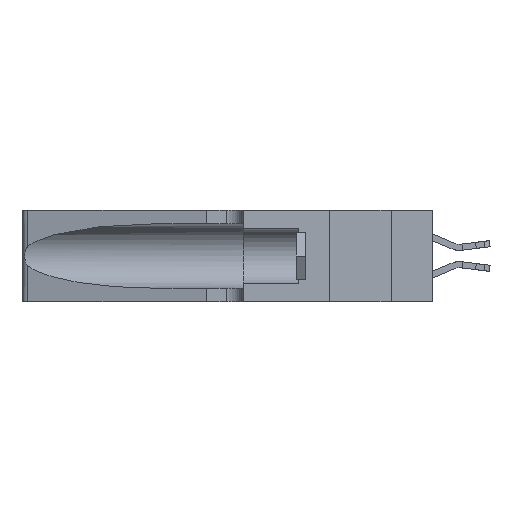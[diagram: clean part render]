
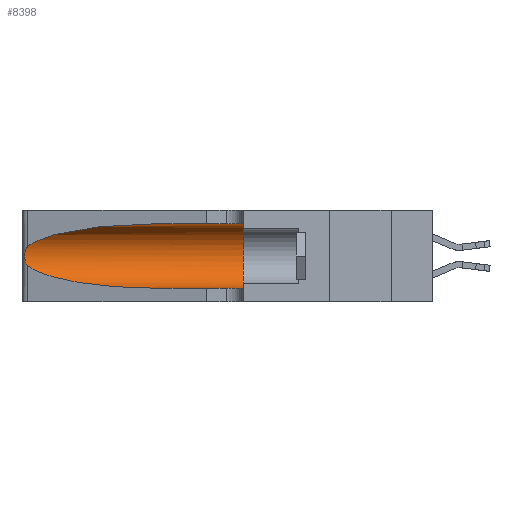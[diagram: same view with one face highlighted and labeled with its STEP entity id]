
A CAD part, left-side view. The second image highlights one B-rep face of the part: STEP entity #8398.
In plain terms, the highlighted cylindrical face has radius 3.308 mm (diameter 6.617 mm), a partial arc.
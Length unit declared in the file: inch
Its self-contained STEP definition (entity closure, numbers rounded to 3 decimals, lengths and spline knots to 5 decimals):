
#707 = CARTESIAN_POINT ( 'NONE',  ( 0.2373, 1.15595, 0.28018 ) ) ;
#922 = VECTOR ( 'NONE', #23108, 39.37008 ) ;
#1194 = CARTESIAN_POINT ( 'NONE',  ( 0.25487, 1.22718, 0.14631 ) ) ;
#1279 = DIRECTION ( 'NONE',  ( 0., 0., 1. ) ) ;
#1360 = ORIENTED_EDGE ( 'NONE', *, *, #14888, .F. ) ;
#1489 = CARTESIAN_POINT ( 'NONE',  ( 0.18966, 0.96281, 0.05475 ) ) ;
#2453 = LINE ( 'NONE', #9547, #922 ) ;
#2675 = CARTESIAN_POINT ( 'NONE',  ( 0.18966, 0.96281, 0.31525 ) ) ;
#3055 = EDGE_CURVE ( 'NONE', #12755, #5751, #14692, .T. ) ;
#3544 = CARTESIAN_POINT ( 'NONE',  ( 0.2373, 1.15595, 0.08982 ) ) ;
#4794 = DIRECTION ( 'NONE',  ( 0., 0., -1. ) ) ;
#4878 = CARTESIAN_POINT ( 'NONE',  ( 0.26075, 1.23896, 0.19203 ) ) ;
#4987 = CARTESIAN_POINT ( 'NONE',  ( 0.1305, 0.72297, 0.05475 ) ) ;
#5050 = CARTESIAN_POINT ( 'NONE',  ( 0.25854, 1.2359, 0.20912 ) ) ;
#5258 = EDGE_CURVE ( 'NONE', #9538, #23373, #2453, .T. ) ;
#5751 = VERTEX_POINT ( 'NONE', #22808 ) ;
#6125 = DIRECTION ( 'NONE',  ( 0., -1., 0. ) ) ;
#6183 = AXIS2_PLACEMENT_3D ( 'NONE', #6926, #8878, #1279 ) ;
#6446 = CARTESIAN_POINT ( 'NONE',  ( 0.1305, 0.35, 0.31525 ) ) ;
#6926 = CARTESIAN_POINT ( 'NONE',  ( 0.1305, 0.35, 0.185 ) ) ;
#7015 = CARTESIAN_POINT ( 'NONE',  ( 0.25856, 1.23593, 0.16098 ) ) ;
#7385 = CARTESIAN_POINT ( 'NONE',  ( 0.1305, 0.72297, 0.05475 ) ) ;
#7929 = CARTESIAN_POINT ( 'NONE',  ( 0.25487, 1.22718, 0.14631 ) ) ;
#8147 = CARTESIAN_POINT ( 'NONE',  ( 0.1305, 0.35, 0.05475 ) ) ;
#8299 = ORIENTED_EDGE ( 'NONE', *, *, #3055, .T. ) ;
#8398 = ADVANCED_FACE ( 'NONE', ( #16688 ), #8464, .F. ) ;
#8464 = CYLINDRICAL_SURFACE ( 'NONE', #13961, 0.13025 ) ;
#8497 = EDGE_CURVE ( 'NONE', #5751, #16210, #12018, .T. ) ;
#8878 = DIRECTION ( 'NONE',  ( 0., 1., 0. ) ) ;
#8970 = CARTESIAN_POINT ( 'NONE',  ( 0.25487, 1.22718, 0.22369 ) ) ;
#9538 = VERTEX_POINT ( 'NONE', #4987 ) ;
#9547 = CARTESIAN_POINT ( 'NONE',  ( 0.1305, 1.61858, 0.05475 ) ) ;
#10218 = CARTESIAN_POINT ( 'NONE',  ( 0.1305, 1.61858, 0.31525 ) ) ;
#10250 = EDGE_CURVE ( 'NONE', #16210, #9538, #10942, .T. ) ;
#10326 = DIRECTION ( 'NONE',  ( 0., -1., 0. ) ) ;
#10418 = CARTESIAN_POINT ( 'NONE',  ( 0.25487, 1.22718, 0.22369 ) ) ;
#10740 = VECTOR ( 'NONE', #6125, 39.37008 ) ;
#10747 = CARTESIAN_POINT ( 'NONE',  ( 0.26017, 1.23833, 0.17102 ) ) ;
#10820 = EDGE_CURVE ( 'NONE', #18392, #23373, #21739, .T. ) ;
#10829 = CARTESIAN_POINT ( 'NONE',  ( 0.25639, 1.23186, 0.15144 ) ) ;
#10942 =( BOUNDED_CURVE ( )  B_SPLINE_CURVE ( 3, ( #12853, #3544, #1489, #7385 ),
 .UNSPECIFIED., .F., .F. ) 
 B_SPLINE_CURVE_WITH_KNOTS ( ( 4, 4 ),
 ( 3.44316, 4.71239 ),
 .UNSPECIFIED. ) 
 CURVE ( )  GEOMETRIC_REPRESENTATION_ITEM ( )  RATIONAL_B_SPLINE_CURVE ( ( 1., 0.87, 0.87, 1. ) ) 
 REPRESENTATION_ITEM ( '' )  );
#12018 = B_SPLINE_CURVE_WITH_KNOTS ( 'NONE', 3,
 ( #8970, #12951, #22551, #16694, #5050, #16612, #4878, #16874, #10747, #7015, #18571, #10829, #24497, #1194 ),
 .UNSPECIFIED., .F., .F.,
 ( 4, 2, 2, 2, 2, 2, 4 ),
 ( 0., 0.00027, 0.00053, 0.00107, 0.0016, 0.00187, 0.00214 ),
 .UNSPECIFIED. ) ;
#12334 = CARTESIAN_POINT ( 'NONE',  ( 0.1305, 1.61858, 0.185 ) ) ;
#12755 = VERTEX_POINT ( 'NONE', #15974 ) ;
#12853 = CARTESIAN_POINT ( 'NONE',  ( 0.25487, 1.22718, 0.14631 ) ) ;
#12951 = CARTESIAN_POINT ( 'NONE',  ( 0.25555, 1.22994, 0.2215 ) ) ;
#13238 = ORIENTED_EDGE ( 'NONE', *, *, #5258, .T. ) ;
#13961 = AXIS2_PLACEMENT_3D ( 'NONE', #12334, #10326, #4794 ) ;
#14692 =( BOUNDED_CURVE ( )  B_SPLINE_CURVE ( 3, ( #18181, #2675, #707, #10418 ),
 .UNSPECIFIED., .F., .F. ) 
 B_SPLINE_CURVE_WITH_KNOTS ( ( 4, 4 ),
 ( 1.5708, 2.84003 ),
 .UNSPECIFIED. ) 
 CURVE ( )  GEOMETRIC_REPRESENTATION_ITEM ( )  RATIONAL_B_SPLINE_CURVE ( ( 1., 0.87, 0.87, 1. ) ) 
 REPRESENTATION_ITEM ( '' )  );
#14888 = EDGE_CURVE ( 'NONE', #12755, #18392, #17419, .T. ) ;
#15974 = CARTESIAN_POINT ( 'NONE',  ( 0.1305, 0.72297, 0.31525 ) ) ;
#16210 = VERTEX_POINT ( 'NONE', #7929 ) ;
#16237 = ORIENTED_EDGE ( 'NONE', *, *, #8497, .T. ) ;
#16612 = CARTESIAN_POINT ( 'NONE',  ( 0.26018, 1.23835, 0.19895 ) ) ;
#16688 = FACE_OUTER_BOUND ( 'NONE', #19490, .T. ) ;
#16694 = CARTESIAN_POINT ( 'NONE',  ( 0.25787, 1.23484, 0.2124 ) ) ;
#16874 = CARTESIAN_POINT ( 'NONE',  ( 0.26075, 1.23896, 0.178 ) ) ;
#17419 = LINE ( 'NONE', #10218, #10740 ) ;
#18181 = CARTESIAN_POINT ( 'NONE',  ( 0.1305, 0.72297, 0.31525 ) ) ;
#18392 = VERTEX_POINT ( 'NONE', #6446 ) ;
#18571 = CARTESIAN_POINT ( 'NONE',  ( 0.25789, 1.23486, 0.15765 ) ) ;
#19490 = EDGE_LOOP ( 'NONE', ( #8299, #16237, #22023, #13238, #24963, #1360 ) ) ;
#21739 = CIRCLE ( 'NONE', #6183, 0.13025 ) ;
#22023 = ORIENTED_EDGE ( 'NONE', *, *, #10250, .T. ) ;
#22551 = CARTESIAN_POINT ( 'NONE',  ( 0.25639, 1.23184, 0.21858 ) ) ;
#22808 = CARTESIAN_POINT ( 'NONE',  ( 0.25487, 1.22718, 0.22369 ) ) ;
#23108 = DIRECTION ( 'NONE',  ( 0., -1., 0. ) ) ;
#23373 = VERTEX_POINT ( 'NONE', #8147 ) ;
#24497 = CARTESIAN_POINT ( 'NONE',  ( 0.25555, 1.22993, 0.14849 ) ) ;
#24963 = ORIENTED_EDGE ( 'NONE', *, *, #10820, .F. ) ;
